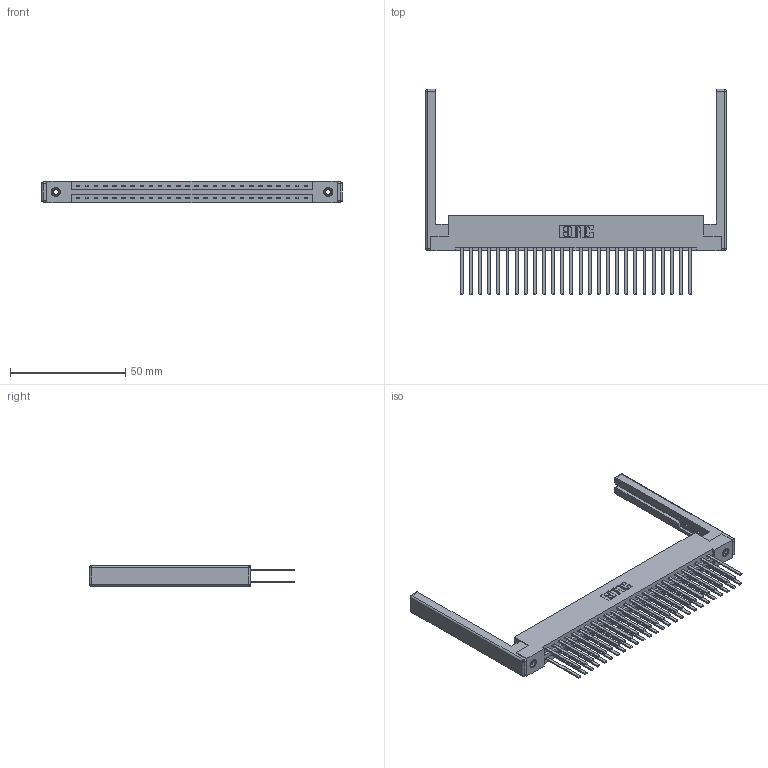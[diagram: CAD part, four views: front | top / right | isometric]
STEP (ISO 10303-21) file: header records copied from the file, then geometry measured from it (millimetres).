
FILE_DESCRIPTION (( 'STEP AP203' ), '1' );
FILE_NAME ('387-052-544-268.STEP', '2019-10-19T03:34:59', ( '' ), ( '' ), 'SwSTEP 2.0', 'SolidWorks 2016', '' );
FILE_SCHEMA (( 'CONFIG_CONTROL_DESIGN' ));
Length unit declared in the file: inch
Products named in the file (5): 307-220-068; 337 Part_Flush Mounting Lugs - 0.156 Dia-TI; 387-052-544-268; 345-250-001_345-250-001-102; 345-292-001_345-293-144
Assembly tree (57 placements, depth 2):
  387-052-544-268
    337 Part_Flush Mounting Lugs - 0.156 Dia-TI
    345-292-001_345-293-144  x52
    345-250-001_345-250-001-102  x2
    307-220-068  x2
Bounding box: 130.45 x 89.03 x 9.4 mm (x, y, z)
Volume: 18649.1 mm3; surface area: 22386 mm2
Topology: 57 solids, 57 shells, 2764 faces, 8137 edges, 5334 vertices
Faces by surface type: plane 1926, cylinder 814, cone 12, sphere 8, torus 4
Entity records: 24804 total; most frequent: CARTESIAN_POINT 4155, ORIENTED_EDGE 4080, DIRECTION 3630, EDGE_CURVE 2040, VECTOR 1866, LINE 1866, VERTEX_POINT 1350, AXIS2_PLACEMENT_3D 882
